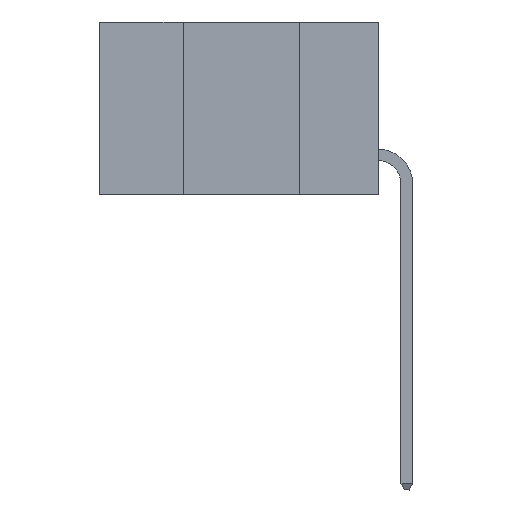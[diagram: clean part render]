
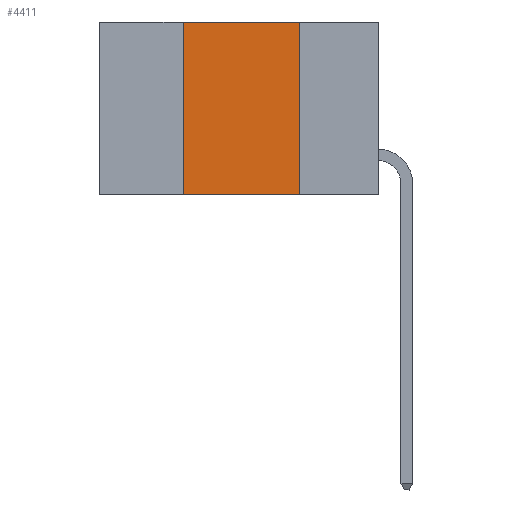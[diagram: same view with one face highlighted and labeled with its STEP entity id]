
A CAD part, left-side view. The second image highlights one B-rep face of the part: STEP entity #4411.
In plain terms, the highlighted planar face has unit normal (-1, 0, 0).
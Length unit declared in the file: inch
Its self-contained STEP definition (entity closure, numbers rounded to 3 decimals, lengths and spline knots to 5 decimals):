
#95 = CARTESIAN_POINT ( 'NONE',  ( 0., 0.42, 0. ) ) ;
#459 = DIRECTION ( 'NONE',  ( 0., 0., -1. ) ) ;
#796 = ORIENTED_EDGE ( 'NONE', *, *, #8723, .F. ) ;
#1194 = CARTESIAN_POINT ( 'NONE',  ( 0., 0.17, -0.37 ) ) ;
#1685 = DIRECTION ( 'NONE',  ( 0., -1., 0. ) ) ;
#1741 = VERTEX_POINT ( 'NONE', #9415 ) ;
#1996 = LINE ( 'NONE', #5131, #5267 ) ;
#2141 = PLANE ( 'NONE',  #9018 ) ;
#2300 = CARTESIAN_POINT ( 'NONE',  ( 0., 0.42, -0.37 ) ) ;
#2657 = VECTOR ( 'NONE', #1685, 39.37008 ) ;
#2661 = VERTEX_POINT ( 'NONE', #6062 ) ;
#3282 = VERTEX_POINT ( 'NONE', #2300 ) ;
#3411 = LINE ( 'NONE', #6372, #2657 ) ;
#3478 = ORIENTED_EDGE ( 'NONE', *, *, #9536, .F. ) ;
#3631 = VERTEX_POINT ( 'NONE', #95 ) ;
#4339 = DIRECTION ( 'NONE',  ( 0., -1., 0. ) ) ;
#4411 = ADVANCED_FACE ( 'NONE', ( #10004 ), #2141, .F. ) ;
#5131 = CARTESIAN_POINT ( 'NONE',  ( 0., 0.6, -0.37 ) ) ;
#5199 = ORIENTED_EDGE ( 'NONE', *, *, #6957, .T. ) ;
#5267 = VECTOR ( 'NONE', #4339, 39.37008 ) ;
#5273 = VECTOR ( 'NONE', #8305, 39.37008 ) ;
#5957 = VECTOR ( 'NONE', #459, 39.37008 ) ;
#6062 = CARTESIAN_POINT ( 'NONE',  ( 0., 0.17, -0.37 ) ) ;
#6372 = CARTESIAN_POINT ( 'NONE',  ( 0., 0.6, 0. ) ) ;
#6822 = LINE ( 'NONE', #9272, #5273 ) ;
#6957 = EDGE_CURVE ( 'NONE', #3282, #2661, #1996, .T. ) ;
#7467 = CARTESIAN_POINT ( 'NONE',  ( 0., 0.6, 0. ) ) ;
#7577 = DIRECTION ( 'NONE',  ( 0., 0., -1. ) ) ;
#8192 = EDGE_CURVE ( 'NONE', #3631, #1741, #3411, .T. ) ;
#8305 = DIRECTION ( 'NONE',  ( 0., 0., 1. ) ) ;
#8370 = DIRECTION ( 'NONE',  ( 1., 0., 0. ) ) ;
#8723 = EDGE_CURVE ( 'NONE', #1741, #2661, #9932, .T. ) ;
#8759 = EDGE_LOOP ( 'NONE', ( #796, #10167, #3478, #5199 ) ) ;
#9018 = AXIS2_PLACEMENT_3D ( 'NONE', #7467, #8370, #7577 ) ;
#9272 = CARTESIAN_POINT ( 'NONE',  ( 0., 0.42, -0.37 ) ) ;
#9415 = CARTESIAN_POINT ( 'NONE',  ( 0., 0.17, 0. ) ) ;
#9536 = EDGE_CURVE ( 'NONE', #3282, #3631, #6822, .T. ) ;
#9932 = LINE ( 'NONE', #1194, #5957 ) ;
#10004 = FACE_OUTER_BOUND ( 'NONE', #8759, .T. ) ;
#10167 = ORIENTED_EDGE ( 'NONE', *, *, #8192, .F. ) ;
